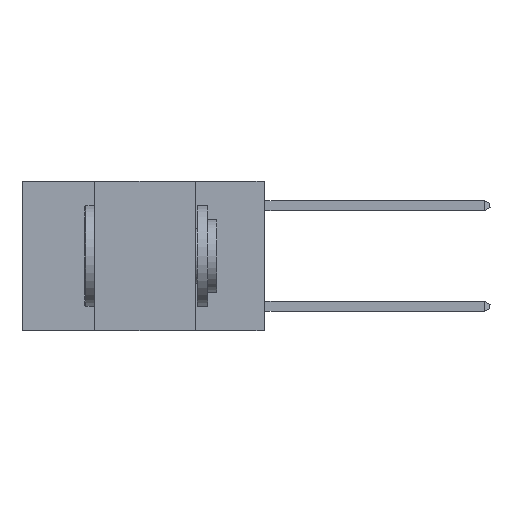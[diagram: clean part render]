
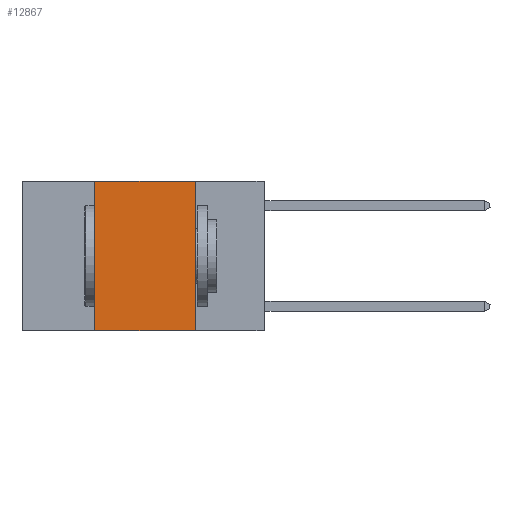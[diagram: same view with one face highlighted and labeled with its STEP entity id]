
A CAD part, left-side view. The second image highlights one B-rep face of the part: STEP entity #12867.
In plain terms, the highlighted planar face has unit normal (-1, 0, 0).
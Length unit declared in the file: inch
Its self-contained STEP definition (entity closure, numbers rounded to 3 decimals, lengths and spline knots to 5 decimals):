
#508 = DIRECTION ( 'NONE',  ( 0., 0., -1. ) ) ;
#1505 = ORIENTED_EDGE ( 'NONE', *, *, #28850, .F. ) ;
#2498 = DIRECTION ( 'NONE',  ( 0., 0., -1. ) ) ;
#4786 = CARTESIAN_POINT ( 'NONE',  ( 0., 0.17, 0. ) ) ;
#4917 = VECTOR ( 'NONE', #10731, 39.37008 ) ;
#5227 = DIRECTION ( 'NONE',  ( 0., -1., 0. ) ) ;
#6082 = DIRECTION ( 'NONE',  ( 0., -1., 0. ) ) ;
#7059 = LINE ( 'NONE', #17047, #17926 ) ;
#7241 = DIRECTION ( 'NONE',  ( 1., 0., 0. ) ) ;
#7685 = CARTESIAN_POINT ( 'NONE',  ( 0., 0.6, -0.37 ) ) ;
#8561 = EDGE_LOOP ( 'NONE', ( #16519, #1505, #16224, #10866 ) ) ;
#8756 = VECTOR ( 'NONE', #5227, 39.37008 ) ;
#10245 = CARTESIAN_POINT ( 'NONE',  ( 0., 0.42, 0. ) ) ;
#10731 = DIRECTION ( 'NONE',  ( 0., 0., 1. ) ) ;
#10866 = ORIENTED_EDGE ( 'NONE', *, *, #14633, .T. ) ;
#10979 = CARTESIAN_POINT ( 'NONE',  ( 0., 0.42, 0. ) ) ;
#12609 = PLANE ( 'NONE',  #20802 ) ;
#12867 = ADVANCED_FACE ( 'NONE', ( #17387 ), #12609, .F. ) ;
#13271 = CARTESIAN_POINT ( 'NONE',  ( 0., 0.6, 0. ) ) ;
#14633 = EDGE_CURVE ( 'NONE', #29467, #19978, #30112, .T. ) ;
#16224 = ORIENTED_EDGE ( 'NONE', *, *, #22604, .F. ) ;
#16519 = ORIENTED_EDGE ( 'NONE', *, *, #19044, .F. ) ;
#17047 = CARTESIAN_POINT ( 'NONE',  ( 0., 0.17, 0. ) ) ;
#17176 = VECTOR ( 'NONE', #6082, 39.37008 ) ;
#17387 = FACE_OUTER_BOUND ( 'NONE', #8561, .T. ) ;
#17778 = LINE ( 'NONE', #10245, #4917 ) ;
#17926 = VECTOR ( 'NONE', #508, 39.37008 ) ;
#18893 = CARTESIAN_POINT ( 'NONE',  ( 0., 0.42, -0.37 ) ) ;
#19044 = EDGE_CURVE ( 'NONE', #21069, #19978, #7059, .T. ) ;
#19978 = VERTEX_POINT ( 'NONE', #29681 ) ;
#20802 = AXIS2_PLACEMENT_3D ( 'NONE', #29659, #7241, #2498 ) ;
#21069 = VERTEX_POINT ( 'NONE', #4786 ) ;
#22604 = EDGE_CURVE ( 'NONE', #29467, #27467, #17778, .T. ) ;
#27467 = VERTEX_POINT ( 'NONE', #10979 ) ;
#28850 = EDGE_CURVE ( 'NONE', #27467, #21069, #30460, .T. ) ;
#29467 = VERTEX_POINT ( 'NONE', #18893 ) ;
#29659 = CARTESIAN_POINT ( 'NONE',  ( 0., 0.6, 0. ) ) ;
#29681 = CARTESIAN_POINT ( 'NONE',  ( 0., 0.17, -0.37 ) ) ;
#30112 = LINE ( 'NONE', #7685, #8756 ) ;
#30460 = LINE ( 'NONE', #13271, #17176 ) ;
